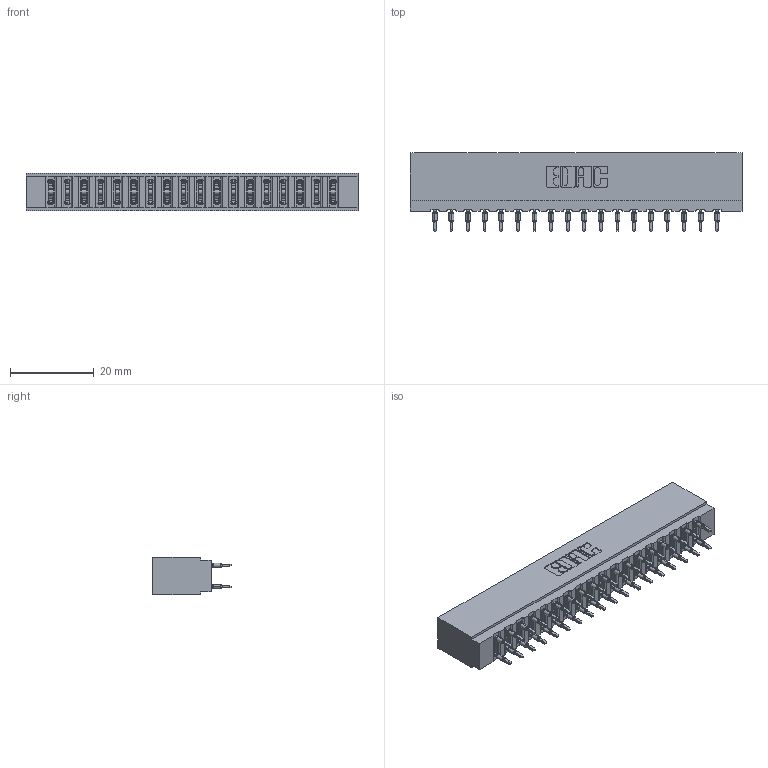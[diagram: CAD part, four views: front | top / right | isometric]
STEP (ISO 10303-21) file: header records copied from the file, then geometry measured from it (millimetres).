
FILE_DESCRIPTION (( 'STEP AP203' ), '1' );
FILE_NAME ('717-036-560-201.STEP', '2026-02-20T17:46:39', ( '' ), ( '' ), 'SwSTEP 2.0', 'SolidWorks 2023', '' );
FILE_SCHEMA (( 'CONFIG_CONTROL_DESIGN' ));
Length unit declared in the file: millimetre
Products named in the file (3): 745-292-001_560; 717 Part_Insulator Option - 06; 717-036-560-201
Assembly tree (37 placements, depth 2):
  717-036-560-201
    717 Part_Insulator Option - 06
    745-292-001_560  x36
Bounding box: 79.2 x 18.78 x 8.89 mm (x, y, z)
Volume: 7094.7 mm3; surface area: 11164.2 mm2
Topology: 37 solids, 37 shells, 3658 faces, 10007 edges, 6358 vertices
Faces by surface type: plane 1908, cylinder 814, bspline 720, torus 216
Entity records: 34428 total; most frequent: CARTESIAN_POINT 6487, ORIENTED_EDGE 5874, DIRECTION 5155, EDGE_CURVE 2937, VECTOR 2639, LINE 2639, VERTEX_POINT 1878, AXIS2_PLACEMENT_3D 1258
